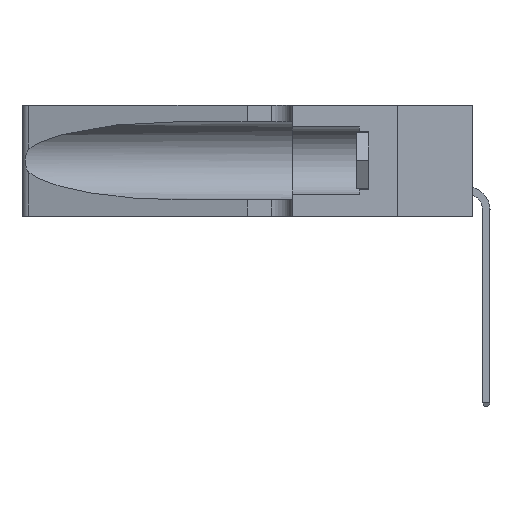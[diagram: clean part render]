
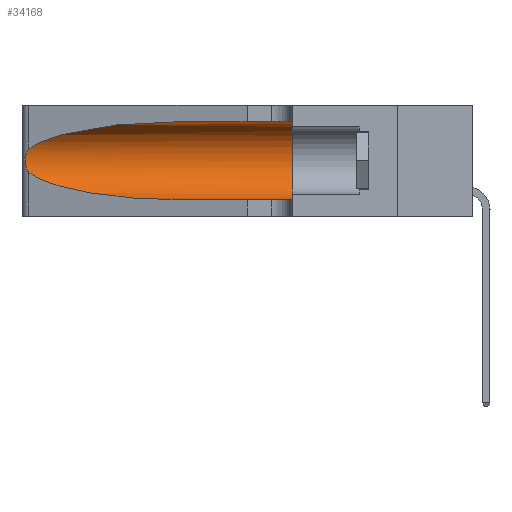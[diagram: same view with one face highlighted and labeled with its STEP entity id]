
A CAD part, left-side view. The second image highlights one B-rep face of the part: STEP entity #34168.
In plain terms, the highlighted cylindrical face has radius 3.308 mm (diameter 6.617 mm), a partial arc.
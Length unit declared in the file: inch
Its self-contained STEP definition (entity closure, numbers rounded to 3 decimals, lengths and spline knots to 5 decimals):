
#320 = CIRCLE ( 'NONE', #24873, 0.13025 ) ;
#1682 = DIRECTION ( 'NONE',  ( 0., -1., 0. ) ) ;
#1887 = CARTESIAN_POINT ( 'NONE',  ( 0.18966, 0.96281, 0.31525 ) ) ;
#2733 = CARTESIAN_POINT ( 'NONE',  ( 0.1305, 0.72297, 0.31525 ) ) ;
#2813 = VERTEX_POINT ( 'NONE', #39211 ) ;
#2866 = CARTESIAN_POINT ( 'NONE',  ( 0.25487, 1.22718, 0.14631 ) ) ;
#3398 = CARTESIAN_POINT ( 'NONE',  ( 0.25487, 1.22718, 0.22369 ) ) ;
#3908 = FACE_OUTER_BOUND ( 'NONE', #26567, .T. ) ;
#5293 = B_SPLINE_CURVE_WITH_KNOTS ( 'NONE', 3,
 ( #3398, #25132, #16173, #12777, #22390, #9471, #6308, #15662, #12511, #19082, #37605, #22005, #18947, #28638 ),
 .UNSPECIFIED., .F., .F.,
 ( 4, 2, 2, 2, 2, 2, 4 ),
 ( 0., 0.00027, 0.00053, 0.00107, 0.0016, 0.00187, 0.00214 ),
 .UNSPECIFIED. ) ;
#5330 = ORIENTED_EDGE ( 'NONE', *, *, #21867, .T. ) ;
#6308 = CARTESIAN_POINT ( 'NONE',  ( 0.26075, 1.23896, 0.19203 ) ) ;
#7962 = CARTESIAN_POINT ( 'NONE',  ( 0.25487, 1.22718, 0.22369 ) ) ;
#8094 = EDGE_CURVE ( 'NONE', #32013, #2813, #320, .T. ) ;
#8503 = CARTESIAN_POINT ( 'NONE',  ( 0.25487, 1.22718, 0.14631 ) ) ;
#9060 = CARTESIAN_POINT ( 'NONE',  ( 0.1305, 0.72297, 0.31525 ) ) ;
#9471 = CARTESIAN_POINT ( 'NONE',  ( 0.26018, 1.23835, 0.19895 ) ) ;
#11253 = DIRECTION ( 'NONE',  ( 0., 0., 1. ) ) ;
#12159 = ORIENTED_EDGE ( 'NONE', *, *, #16527, .F. ) ;
#12511 = CARTESIAN_POINT ( 'NONE',  ( 0.26017, 1.23833, 0.17102 ) ) ;
#12722 = ORIENTED_EDGE ( 'NONE', *, *, #30496, .T. ) ;
#12777 = CARTESIAN_POINT ( 'NONE',  ( 0.25787, 1.23484, 0.2124 ) ) ;
#14097 = VERTEX_POINT ( 'NONE', #8503 ) ;
#14151 = CARTESIAN_POINT ( 'NONE',  ( 0.1305, 0.72297, 0.05475 ) ) ;
#14354 = ORIENTED_EDGE ( 'NONE', *, *, #8094, .F. ) ;
#14470 = CARTESIAN_POINT ( 'NONE',  ( 0.1305, 1.61858, 0.31525 ) ) ;
#14639 = DIRECTION ( 'NONE',  ( 0., -1., 0. ) ) ;
#15662 = CARTESIAN_POINT ( 'NONE',  ( 0.26075, 1.23896, 0.178 ) ) ;
#16173 = CARTESIAN_POINT ( 'NONE',  ( 0.25639, 1.23184, 0.21858 ) ) ;
#16527 = EDGE_CURVE ( 'NONE', #29265, #32013, #35901, .T. ) ;
#17415 = CARTESIAN_POINT ( 'NONE',  ( 0.1305, 0.35, 0.185 ) ) ;
#17584 = ORIENTED_EDGE ( 'NONE', *, *, #21097, .T. ) ;
#18217 = VECTOR ( 'NONE', #1682, 39.37008 ) ;
#18283 = CARTESIAN_POINT ( 'NONE',  ( 0.2373, 1.15595, 0.08982 ) ) ;
#18947 = CARTESIAN_POINT ( 'NONE',  ( 0.25555, 1.22993, 0.14849 ) ) ;
#19082 = CARTESIAN_POINT ( 'NONE',  ( 0.25856, 1.23593, 0.16098 ) ) ;
#21097 = EDGE_CURVE ( 'NONE', #28898, #14097, #5293, .T. ) ;
#21867 = EDGE_CURVE ( 'NONE', #29157, #2813, #36843, .T. ) ;
#22005 = CARTESIAN_POINT ( 'NONE',  ( 0.25639, 1.23186, 0.15144 ) ) ;
#22390 = CARTESIAN_POINT ( 'NONE',  ( 0.25854, 1.2359, 0.20912 ) ) ;
#22726 = CARTESIAN_POINT ( 'NONE',  ( 0.1305, 1.61858, 0.185 ) ) ;
#24873 = AXIS2_PLACEMENT_3D ( 'NONE', #17415, #39371, #11253 ) ;
#25132 = CARTESIAN_POINT ( 'NONE',  ( 0.25555, 1.22994, 0.2215 ) ) ;
#26567 = EDGE_LOOP ( 'NONE', ( #12722, #17584, #32912, #5330, #14354, #12159 ) ) ;
#27174 = CARTESIAN_POINT ( 'NONE',  ( 0.2373, 1.15595, 0.28018 ) ) ;
#28638 = CARTESIAN_POINT ( 'NONE',  ( 0.25487, 1.22718, 0.14631 ) ) ;
#28652 = CARTESIAN_POINT ( 'NONE',  ( 0.25487, 1.22718, 0.22369 ) ) ;
#28898 = VERTEX_POINT ( 'NONE', #28652 ) ;
#29157 = VERTEX_POINT ( 'NONE', #14151 ) ;
#29265 = VERTEX_POINT ( 'NONE', #9060 ) ;
#30496 = EDGE_CURVE ( 'NONE', #29265, #28898, #31420, .T. ) ;
#30662 = AXIS2_PLACEMENT_3D ( 'NONE', #22726, #14639, #36552 ) ;
#30728 = CARTESIAN_POINT ( 'NONE',  ( 0.1305, 0.72297, 0.05475 ) ) ;
#31420 =( BOUNDED_CURVE ( )  B_SPLINE_CURVE ( 3, ( #2733, #1887, #27174, #7962 ),
 .UNSPECIFIED., .F., .F. ) 
 B_SPLINE_CURVE_WITH_KNOTS ( ( 4, 4 ),
 ( 1.5708, 2.84003 ),
 .UNSPECIFIED. ) 
 CURVE ( )  GEOMETRIC_REPRESENTATION_ITEM ( )  RATIONAL_B_SPLINE_CURVE ( ( 1., 0.87, 0.87, 1. ) ) 
 REPRESENTATION_ITEM ( '' )  );
#32013 = VERTEX_POINT ( 'NONE', #34232 ) ;
#32665 = EDGE_CURVE ( 'NONE', #14097, #29157, #40033, .T. ) ;
#32847 = CYLINDRICAL_SURFACE ( 'NONE', #30662, 0.13025 ) ;
#32912 = ORIENTED_EDGE ( 'NONE', *, *, #32665, .T. ) ;
#34168 = ADVANCED_FACE ( 'NONE', ( #3908 ), #32847, .F. ) ;
#34232 = CARTESIAN_POINT ( 'NONE',  ( 0.1305, 0.35, 0.31525 ) ) ;
#34256 = CARTESIAN_POINT ( 'NONE',  ( 0.18966, 0.96281, 0.05475 ) ) ;
#35901 = LINE ( 'NONE', #14470, #37410 ) ;
#36552 = DIRECTION ( 'NONE',  ( 0., 0., -1. ) ) ;
#36660 = DIRECTION ( 'NONE',  ( 0., -1., 0. ) ) ;
#36843 = LINE ( 'NONE', #38892, #18217 ) ;
#37410 = VECTOR ( 'NONE', #36660, 39.37008 ) ;
#37605 = CARTESIAN_POINT ( 'NONE',  ( 0.25789, 1.23486, 0.15765 ) ) ;
#38892 = CARTESIAN_POINT ( 'NONE',  ( 0.1305, 1.61858, 0.05475 ) ) ;
#39211 = CARTESIAN_POINT ( 'NONE',  ( 0.1305, 0.35, 0.05475 ) ) ;
#39371 = DIRECTION ( 'NONE',  ( 0., 1., 0. ) ) ;
#40033 =( BOUNDED_CURVE ( )  B_SPLINE_CURVE ( 3, ( #2866, #18283, #34256, #30728 ),
 .UNSPECIFIED., .F., .F. ) 
 B_SPLINE_CURVE_WITH_KNOTS ( ( 4, 4 ),
 ( 3.44316, 4.71239 ),
 .UNSPECIFIED. ) 
 CURVE ( )  GEOMETRIC_REPRESENTATION_ITEM ( )  RATIONAL_B_SPLINE_CURVE ( ( 1., 0.87, 0.87, 1. ) ) 
 REPRESENTATION_ITEM ( '' )  );
